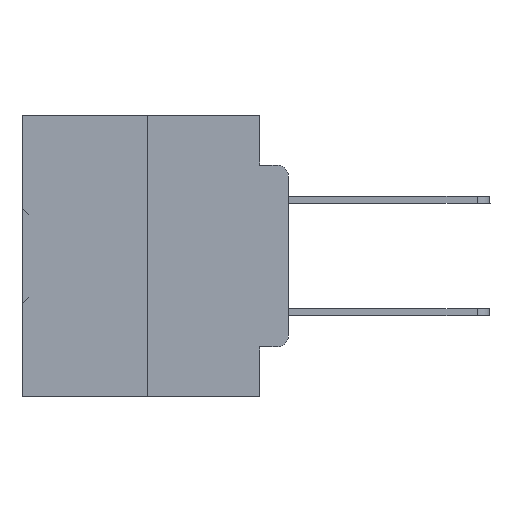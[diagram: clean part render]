
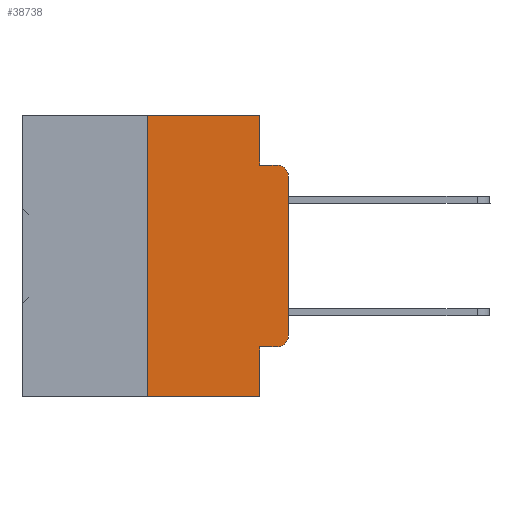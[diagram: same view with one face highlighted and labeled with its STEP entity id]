
A CAD part, left-side view. The second image highlights one B-rep face of the part: STEP entity #38738.
In plain terms, the highlighted planar face has unit normal (-1, 0, 0).
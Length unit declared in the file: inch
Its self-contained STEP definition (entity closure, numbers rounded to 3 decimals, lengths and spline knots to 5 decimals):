
#420 = CARTESIAN_POINT ( 'NONE',  ( 0., 0.051, 0. ) ) ;
#525 = LINE ( 'NONE', #23723, #32506 ) ;
#678 = ORIENTED_EDGE ( 'NONE', *, *, #10852, .F. ) ;
#749 = VERTEX_POINT ( 'NONE', #35480 ) ;
#1090 = PLANE ( 'NONE',  #3510 ) ;
#1095 = CARTESIAN_POINT ( 'NONE',  ( 0., 0.02, -0.3915 ) ) ;
#1222 = DIRECTION ( 'NONE',  ( 1., 0., 0. ) ) ;
#1673 = CARTESIAN_POINT ( 'NONE',  ( 0., 0.051, -0.0885 ) ) ;
#1758 = EDGE_LOOP ( 'NONE', ( #29771, #24455, #32653, #678, #27365, #3586, #23065, #15831, #2169, #26893 ) ) ;
#1979 = VERTEX_POINT ( 'NONE', #1673 ) ;
#2145 = DIRECTION ( 'NONE',  ( 0., -1., 0. ) ) ;
#2169 = ORIENTED_EDGE ( 'NONE', *, *, #36474, .T. ) ;
#2721 = DIRECTION ( 'NONE',  ( 0., 0., -1. ) ) ;
#3161 = VERTEX_POINT ( 'NONE', #20156 ) ;
#3329 = CIRCLE ( 'NONE', #20858, 0.02 ) ;
#3510 = AXIS2_PLACEMENT_3D ( 'NONE', #19904, #1222, #22974 ) ;
#3527 = DIRECTION ( 'NONE',  ( 0., 0., 1. ) ) ;
#3586 = ORIENTED_EDGE ( 'NONE', *, *, #8759, .F. ) ;
#3887 = DIRECTION ( 'NONE',  ( 0., 0., 1. ) ) ;
#4210 = DIRECTION ( 'NONE',  ( 0., 0., -1. ) ) ;
#6014 = DIRECTION ( 'NONE',  ( 0., -1., 0. ) ) ;
#6410 = DIRECTION ( 'NONE',  ( 0., 0., -1. ) ) ;
#7551 = AXIS2_PLACEMENT_3D ( 'NONE', #1095, #22857, #4210 ) ;
#8161 = LINE ( 'NONE', #10165, #31891 ) ;
#8323 = CARTESIAN_POINT ( 'NONE',  ( 0., 0., -0.3915 ) ) ;
#8487 = LINE ( 'NONE', #420, #33180 ) ;
#8759 = EDGE_CURVE ( 'NONE', #17462, #39769, #8161, .T. ) ;
#10165 = CARTESIAN_POINT ( 'NONE',  ( 0., 0.25, 0. ) ) ;
#10852 = EDGE_CURVE ( 'NONE', #16133, #1979, #8487, .T. ) ;
#11653 = DIRECTION ( 'NONE',  ( 0., -1., 0. ) ) ;
#12968 = EDGE_CURVE ( 'NONE', #1979, #26285, #525, .T. ) ;
#13264 = VERTEX_POINT ( 'NONE', #28279 ) ;
#15320 = CARTESIAN_POINT ( 'NONE',  ( 0., 0.473, -0.5 ) ) ;
#15365 = LINE ( 'NONE', #34542, #23556 ) ;
#15831 = ORIENTED_EDGE ( 'NONE', *, *, #38512, .F. ) ;
#15964 = FACE_OUTER_BOUND ( 'NONE', #1758, .T. ) ;
#16133 = VERTEX_POINT ( 'NONE', #35181 ) ;
#16510 = CARTESIAN_POINT ( 'NONE',  ( 0., 0.25, -0.5 ) ) ;
#17462 = VERTEX_POINT ( 'NONE', #16510 ) ;
#18723 = EDGE_CURVE ( 'NONE', #39769, #16133, #38546, .T. ) ;
#19081 = DIRECTION ( 'NONE',  ( 0., 0., -1. ) ) ;
#19904 = CARTESIAN_POINT ( 'NONE',  ( 0., 0.473, 0. ) ) ;
#20156 = CARTESIAN_POINT ( 'NONE',  ( 0., 0.051, -0.5 ) ) ;
#20858 = AXIS2_PLACEMENT_3D ( 'NONE', #39774, #21394, #2721 ) ;
#21288 = EDGE_CURVE ( 'NONE', #25188, #26285, #3329, .T. ) ;
#21394 = DIRECTION ( 'NONE',  ( -1., 0., 0. ) ) ;
#22613 = DIRECTION ( 'NONE',  ( 0., -1., 0. ) ) ;
#22857 = DIRECTION ( 'NONE',  ( -1., 0., 0. ) ) ;
#22974 = DIRECTION ( 'NONE',  ( 0., 0., -1. ) ) ;
#23065 = ORIENTED_EDGE ( 'NONE', *, *, #34169, .T. ) ;
#23141 = VECTOR ( 'NONE', #6410, 39.37008 ) ;
#23321 = EDGE_CURVE ( 'NONE', #30014, #25188, #15365, .T. ) ;
#23556 = VECTOR ( 'NONE', #3527, 39.37008 ) ;
#23723 = CARTESIAN_POINT ( 'NONE',  ( 0., 0.051, -0.0885 ) ) ;
#24455 = ORIENTED_EDGE ( 'NONE', *, *, #21288, .T. ) ;
#25188 = VERTEX_POINT ( 'NONE', #37663 ) ;
#26285 = VERTEX_POINT ( 'NONE', #33561 ) ;
#26893 = ORIENTED_EDGE ( 'NONE', *, *, #34402, .T. ) ;
#27365 = ORIENTED_EDGE ( 'NONE', *, *, #18723, .F. ) ;
#27962 = LINE ( 'NONE', #36332, #36186 ) ;
#28279 = CARTESIAN_POINT ( 'NONE',  ( 0., 0.051, -0.4115 ) ) ;
#29771 = ORIENTED_EDGE ( 'NONE', *, *, #23321, .T. ) ;
#30014 = VERTEX_POINT ( 'NONE', #8323 ) ;
#30320 = CARTESIAN_POINT ( 'NONE',  ( 0., 0.25, 0. ) ) ;
#30365 = VECTOR ( 'NONE', #22613, 39.37008 ) ;
#31334 = LINE ( 'NONE', #37262, #23141 ) ;
#31891 = VECTOR ( 'NONE', #3887, 39.37008 ) ;
#32506 = VECTOR ( 'NONE', #2145, 39.37008 ) ;
#32653 = ORIENTED_EDGE ( 'NONE', *, *, #12968, .F. ) ;
#33180 = VECTOR ( 'NONE', #19081, 39.37008 ) ;
#33561 = CARTESIAN_POINT ( 'NONE',  ( 0., 0.02, -0.0885 ) ) ;
#34169 = EDGE_CURVE ( 'NONE', #17462, #3161, #39253, .T. ) ;
#34402 = EDGE_CURVE ( 'NONE', #749, #30014, #36836, .T. ) ;
#34542 = CARTESIAN_POINT ( 'NONE',  ( 0., 0., 0. ) ) ;
#35181 = CARTESIAN_POINT ( 'NONE',  ( 0., 0.051, 0. ) ) ;
#35480 = CARTESIAN_POINT ( 'NONE',  ( 0., 0.02, -0.4115 ) ) ;
#36186 = VECTOR ( 'NONE', #11653, 39.37008 ) ;
#36332 = CARTESIAN_POINT ( 'NONE',  ( 0., 0.051, -0.4115 ) ) ;
#36474 = EDGE_CURVE ( 'NONE', #13264, #749, #27962, .T. ) ;
#36836 = CIRCLE ( 'NONE', #7551, 0.02 ) ;
#37262 = CARTESIAN_POINT ( 'NONE',  ( 0., 0.051, 0. ) ) ;
#37663 = CARTESIAN_POINT ( 'NONE',  ( 0., 0., -0.1085 ) ) ;
#37937 = CARTESIAN_POINT ( 'NONE',  ( 0., 0.473, 0. ) ) ;
#38283 = VECTOR ( 'NONE', #6014, 39.37008 ) ;
#38512 = EDGE_CURVE ( 'NONE', #13264, #3161, #31334, .T. ) ;
#38546 = LINE ( 'NONE', #37937, #30365 ) ;
#38738 = ADVANCED_FACE ( 'NONE', ( #15964 ), #1090, .F. ) ;
#39253 = LINE ( 'NONE', #15320, #38283 ) ;
#39769 = VERTEX_POINT ( 'NONE', #30320 ) ;
#39774 = CARTESIAN_POINT ( 'NONE',  ( 0., 0.02, -0.1085 ) ) ;
